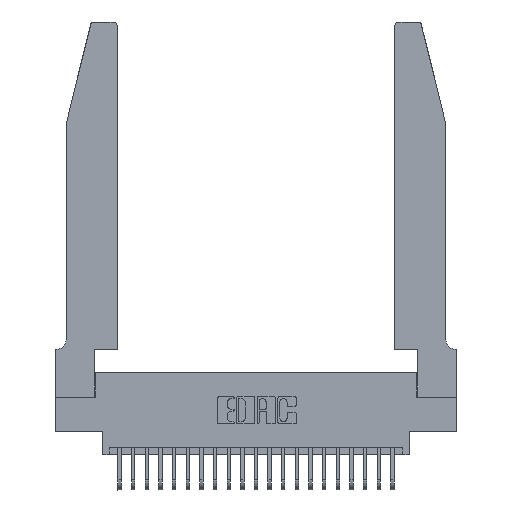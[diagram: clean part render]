
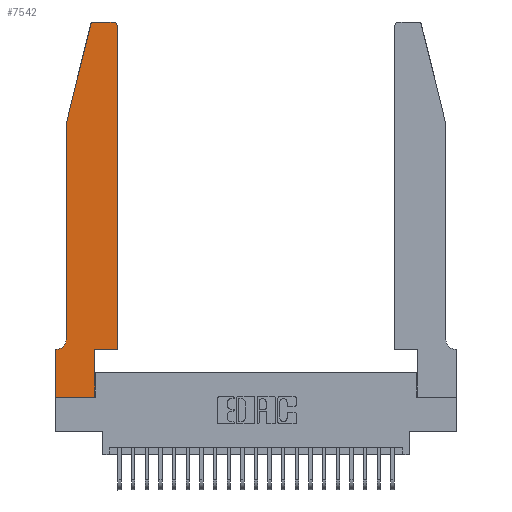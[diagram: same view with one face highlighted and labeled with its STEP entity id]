
A CAD part, top view. The second image highlights one B-rep face of the part: STEP entity #7542.
In plain terms, the highlighted planar face has unit normal (0, 0, 1).
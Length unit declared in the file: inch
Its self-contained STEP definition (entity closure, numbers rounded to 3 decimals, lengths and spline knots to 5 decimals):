
#249 = VERTEX_POINT ( 'NONE', #3954 ) ;
#259 = DIRECTION ( 'NONE',  ( 1., 0., 0. ) ) ;
#995 = EDGE_CURVE ( 'NONE', #11500, #17382, #18611, .T. ) ;
#1196 = EDGE_CURVE ( 'NONE', #249, #7881, #23538, .T. ) ;
#1433 = VECTOR ( 'NONE', #12975, 39.37008 ) ;
#1509 = CARTESIAN_POINT ( 'NONE',  ( 0., 0., 0.37 ) ) ;
#2209 = CARTESIAN_POINT ( 'NONE',  ( 0.4505, 0.35, 0.37 ) ) ;
#2300 = CIRCLE ( 'NONE', #21188, 0.07 ) ;
#3070 = VECTOR ( 'NONE', #22257, 39.37008 ) ;
#3303 = LINE ( 'NONE', #19317, #17409 ) ;
#3471 = LINE ( 'NONE', #18989, #7909 ) ;
#3901 = EDGE_CURVE ( 'NONE', #11244, #16648, #8210, .T. ) ;
#3954 = CARTESIAN_POINT ( 'NONE',  ( 0.2865, 0., 0.37 ) ) ;
#4004 = VECTOR ( 'NONE', #8638, 39.37008 ) ;
#4039 = CIRCLE ( 'NONE', #6952, 0.03 ) ;
#4486 = VECTOR ( 'NONE', #20397, 39.37008 ) ;
#4719 = CARTESIAN_POINT ( 'NONE',  ( 0., 0., 0.37 ) ) ;
#4731 = ORIENTED_EDGE ( 'NONE', *, *, #3901, .T. ) ;
#4842 = DIRECTION ( 'NONE',  ( 0., 0., -1. ) ) ;
#5011 = CIRCLE ( 'NONE', #9840, 0.03 ) ;
#5364 = LINE ( 'NONE', #4719, #15149 ) ;
#5918 = ORIENTED_EDGE ( 'NONE', *, *, #8881, .T. ) ;
#6091 = VERTEX_POINT ( 'NONE', #23408 ) ;
#6268 = DIRECTION ( 'NONE',  ( 0., -1., 0. ) ) ;
#6311 = DIRECTION ( 'NONE',  ( 0., 0., 1. ) ) ;
#6511 = ORIENTED_EDGE ( 'NONE', *, *, #1196, .T. ) ;
#6896 = EDGE_CURVE ( 'NONE', #12488, #6091, #22425, .T. ) ;
#6952 = AXIS2_PLACEMENT_3D ( 'NONE', #17261, #6311, #19025 ) ;
#7542 = ADVANCED_FACE ( 'NONE', ( #20453 ), #20287, .T. ) ;
#7627 = CARTESIAN_POINT ( 'NONE',  ( 0.0755, 2., 0.37 ) ) ;
#7641 = CARTESIAN_POINT ( 'NONE',  ( 0.4205, 2.72, 0.37 ) ) ;
#7757 = CARTESIAN_POINT ( 'NONE',  ( 0., 0.35, 0.37 ) ) ;
#7866 = CARTESIAN_POINT ( 'NONE',  ( 0.0755, 2., 0.37 ) ) ;
#7881 = VERTEX_POINT ( 'NONE', #12200 ) ;
#7909 = VECTOR ( 'NONE', #6268, 39.37008 ) ;
#8210 = LINE ( 'NONE', #11137, #1433 ) ;
#8462 = EDGE_CURVE ( 'NONE', #23053, #20078, #3303, .T. ) ;
#8638 = DIRECTION ( 'NONE',  ( -1., 0., 0. ) ) ;
#8653 = CARTESIAN_POINT ( 'NONE',  ( 0.0055, 0.35, 0.37 ) ) ;
#8881 = EDGE_CURVE ( 'NONE', #7881, #11244, #22078, .T. ) ;
#9510 = DIRECTION ( 'NONE',  ( 1., 0., 0. ) ) ;
#9840 = AXIS2_PLACEMENT_3D ( 'NONE', #7641, #20262, #9510 ) ;
#10058 = CARTESIAN_POINT ( 'NONE',  ( 0., 0.35, 0.37 ) ) ;
#10316 = EDGE_LOOP ( 'NONE', ( #11147, #20145, #20748, #15396, #14268, #13128, #17376, #20944, #6511, #5918, #4731, #18743 ) ) ;
#11137 = CARTESIAN_POINT ( 'NONE',  ( 0.4505, 0.35, 0.37 ) ) ;
#11147 = ORIENTED_EDGE ( 'NONE', *, *, #8462, .T. ) ;
#11244 = VERTEX_POINT ( 'NONE', #13450 ) ;
#11317 = AXIS2_PLACEMENT_3D ( 'NONE', #7757, #11413, #259 ) ;
#11413 = DIRECTION ( 'NONE',  ( 0., 0., 1. ) ) ;
#11500 = VERTEX_POINT ( 'NONE', #8653 ) ;
#12200 = CARTESIAN_POINT ( 'NONE',  ( 0.2865, 0.35, 0.37 ) ) ;
#12488 = VERTEX_POINT ( 'NONE', #22854 ) ;
#12975 = DIRECTION ( 'NONE',  ( 0., 1., 0. ) ) ;
#13128 = ORIENTED_EDGE ( 'NONE', *, *, #995, .T. ) ;
#13450 = CARTESIAN_POINT ( 'NONE',  ( 0.4505, 0.35, 0.37 ) ) ;
#13713 = VECTOR ( 'NONE', #15131, 39.37008 ) ;
#14268 = ORIENTED_EDGE ( 'NONE', *, *, #15828, .T. ) ;
#14875 = LINE ( 'NONE', #7627, #4486 ) ;
#15131 = DIRECTION ( 'NONE',  ( 1., 0., 0. ) ) ;
#15149 = VECTOR ( 'NONE', #17554, 39.37008 ) ;
#15396 = ORIENTED_EDGE ( 'NONE', *, *, #20989, .T. ) ;
#15519 = VERTEX_POINT ( 'NONE', #21924 ) ;
#15828 = EDGE_CURVE ( 'NONE', #15519, #11500, #2300, .T. ) ;
#15862 = CARTESIAN_POINT ( 'NONE',  ( 0.0055, 0.42, 0.37 ) ) ;
#16245 = EDGE_CURVE ( 'NONE', #20078, #12488, #4039, .T. ) ;
#16648 = VERTEX_POINT ( 'NONE', #20292 ) ;
#17261 = CARTESIAN_POINT ( 'NONE',  ( 0.284, 2.72, 0.37 ) ) ;
#17376 = ORIENTED_EDGE ( 'NONE', *, *, #23468, .T. ) ;
#17382 = VERTEX_POINT ( 'NONE', #10058 ) ;
#17409 = VECTOR ( 'NONE', #21106, 39.37008 ) ;
#17554 = DIRECTION ( 'NONE',  ( 1., 0., 0. ) ) ;
#17662 = DIRECTION ( 'NONE',  ( -1., 0., 0. ) ) ;
#17757 = CARTESIAN_POINT ( 'NONE',  ( 0.284, 2.75, 0.37 ) ) ;
#18317 = VERTEX_POINT ( 'NONE', #1509 ) ;
#18611 = LINE ( 'NONE', #21344, #4004 ) ;
#18743 = ORIENTED_EDGE ( 'NONE', *, *, #22289, .T. ) ;
#18877 = VECTOR ( 'NONE', #21616, 39.37008 ) ;
#18989 = CARTESIAN_POINT ( 'NONE',  ( 0., 0., 0.37 ) ) ;
#19025 = DIRECTION ( 'NONE',  ( 1., 0., 0. ) ) ;
#19317 = CARTESIAN_POINT ( 'NONE',  ( 0.2605, 2.75, 0.37 ) ) ;
#20078 = VERTEX_POINT ( 'NONE', #17757 ) ;
#20145 = ORIENTED_EDGE ( 'NONE', *, *, #16245, .T. ) ;
#20262 = DIRECTION ( 'NONE',  ( 0., 0., 1. ) ) ;
#20287 = PLANE ( 'NONE',  #11317 ) ;
#20292 = CARTESIAN_POINT ( 'NONE',  ( 0.4505, 2.72, 0.37 ) ) ;
#20397 = DIRECTION ( 'NONE',  ( 0., -1., 0. ) ) ;
#20453 = FACE_OUTER_BOUND ( 'NONE', #10316, .T. ) ;
#20748 = ORIENTED_EDGE ( 'NONE', *, *, #6896, .T. ) ;
#20776 = CARTESIAN_POINT ( 'NONE',  ( 0.4205, 2.75, 0.37 ) ) ;
#20944 = ORIENTED_EDGE ( 'NONE', *, *, #21171, .T. ) ;
#20989 = EDGE_CURVE ( 'NONE', #6091, #15519, #14875, .T. ) ;
#21106 = DIRECTION ( 'NONE',  ( -1., 0., 0. ) ) ;
#21171 = EDGE_CURVE ( 'NONE', #18317, #249, #5364, .T. ) ;
#21188 = AXIS2_PLACEMENT_3D ( 'NONE', #15862, #4842, #17662 ) ;
#21344 = CARTESIAN_POINT ( 'NONE',  ( 0.0755, 0.35, 0.37 ) ) ;
#21616 = DIRECTION ( 'NONE',  ( 0., 1., 0. ) ) ;
#21924 = CARTESIAN_POINT ( 'NONE',  ( 0.0755, 0.42, 0.37 ) ) ;
#22078 = LINE ( 'NONE', #2209, #13713 ) ;
#22097 = CARTESIAN_POINT ( 'NONE',  ( 0.2865, 0.35, 0.37 ) ) ;
#22257 = DIRECTION ( 'NONE',  ( -0.239, -0.971, 0. ) ) ;
#22289 = EDGE_CURVE ( 'NONE', #16648, #23053, #5011, .T. ) ;
#22425 = LINE ( 'NONE', #7866, #3070 ) ;
#22854 = CARTESIAN_POINT ( 'NONE',  ( 0.25487, 2.72718, 0.37 ) ) ;
#23053 = VERTEX_POINT ( 'NONE', #20776 ) ;
#23408 = CARTESIAN_POINT ( 'NONE',  ( 0.0755, 2., 0.37 ) ) ;
#23468 = EDGE_CURVE ( 'NONE', #17382, #18317, #3471, .T. ) ;
#23538 = LINE ( 'NONE', #22097, #18877 ) ;
